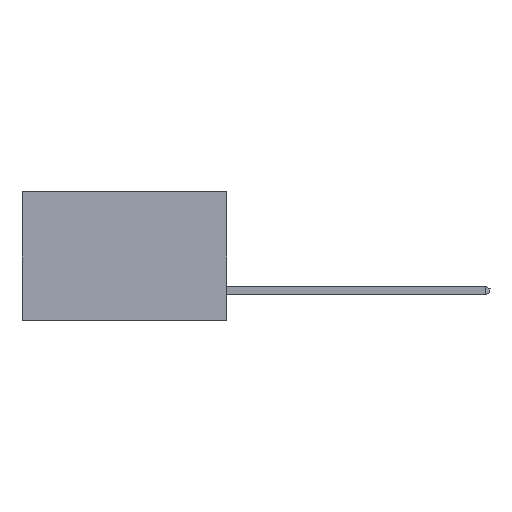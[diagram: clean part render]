
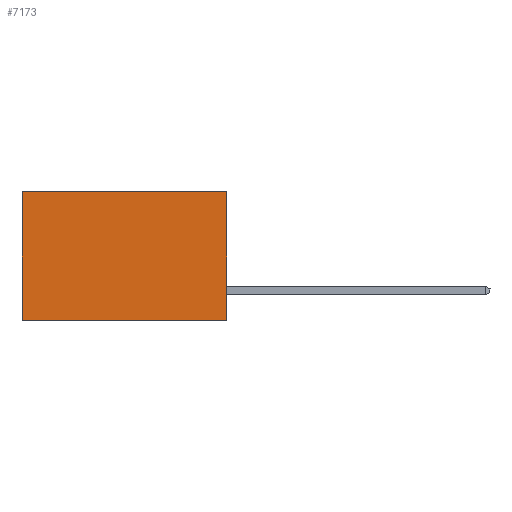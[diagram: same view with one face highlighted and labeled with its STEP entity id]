
A CAD part, left-side view. The second image highlights one B-rep face of the part: STEP entity #7173.
In plain terms, the highlighted planar face has unit normal (-1, 0, 0).
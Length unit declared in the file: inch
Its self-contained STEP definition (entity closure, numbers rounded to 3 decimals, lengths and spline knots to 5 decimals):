
#191 = DIRECTION ( 'NONE',  ( 0., 0., -1. ) ) ;
#784 = ORIENTED_EDGE ( 'NONE', *, *, #5663, .F. ) ;
#1649 = EDGE_CURVE ( 'NONE', #17510, #7373, #10365, .T. ) ;
#2158 = CARTESIAN_POINT ( 'NONE',  ( 0.277, 0., 0. ) ) ;
#2468 = LINE ( 'NONE', #11573, #13204 ) ;
#2965 = DIRECTION ( 'NONE',  ( 0., 1., 0. ) ) ;
#3999 = VECTOR ( 'NONE', #13359, 39.37008 ) ;
#4434 = LINE ( 'NONE', #2158, #3999 ) ;
#4479 = ORIENTED_EDGE ( 'NONE', *, *, #17605, .T. ) ;
#4794 = CARTESIAN_POINT ( 'NONE',  ( 0.277, 0., -0.37 ) ) ;
#5663 = EDGE_CURVE ( 'NONE', #14121, #17510, #2468, .T. ) ;
#7173 = ADVANCED_FACE ( 'NONE', ( #14217 ), #11836, .F. ) ;
#7373 = VERTEX_POINT ( 'NONE', #9023 ) ;
#8032 = EDGE_LOOP ( 'NONE', ( #16727, #12455, #784, #4479 ) ) ;
#9023 = CARTESIAN_POINT ( 'NONE',  ( 0.277, 0.59, -0.37 ) ) ;
#9721 = AXIS2_PLACEMENT_3D ( 'NONE', #12255, #11832, #11819 ) ;
#10365 = LINE ( 'NONE', #4794, #13638 ) ;
#11429 = CARTESIAN_POINT ( 'NONE',  ( 0.277, 0., 0. ) ) ;
#11532 = CARTESIAN_POINT ( 'NONE',  ( 0.277, 0.59, 0. ) ) ;
#11573 = CARTESIAN_POINT ( 'NONE',  ( 0.277, 0., -0.37 ) ) ;
#11819 = DIRECTION ( 'NONE',  ( 0., 0., -1. ) ) ;
#11832 = DIRECTION ( 'NONE',  ( 1., 0., 0. ) ) ;
#11836 = PLANE ( 'NONE',  #9721 ) ;
#11979 = VECTOR ( 'NONE', #191, 39.37008 ) ;
#12255 = CARTESIAN_POINT ( 'NONE',  ( 0.277, 0., -0.37 ) ) ;
#12455 = ORIENTED_EDGE ( 'NONE', *, *, #1649, .F. ) ;
#12848 = CARTESIAN_POINT ( 'NONE',  ( 0.277, 0.59, -0.37 ) ) ;
#13204 = VECTOR ( 'NONE', #14391, 39.37008 ) ;
#13359 = DIRECTION ( 'NONE',  ( 0., 1., 0. ) ) ;
#13405 = VERTEX_POINT ( 'NONE', #11532 ) ;
#13638 = VECTOR ( 'NONE', #2965, 39.37008 ) ;
#14121 = VERTEX_POINT ( 'NONE', #11429 ) ;
#14217 = FACE_OUTER_BOUND ( 'NONE', #8032, .T. ) ;
#14391 = DIRECTION ( 'NONE',  ( 0., 0., -1. ) ) ;
#15617 = LINE ( 'NONE', #12848, #11979 ) ;
#15900 = EDGE_CURVE ( 'NONE', #13405, #7373, #15617, .T. ) ;
#16727 = ORIENTED_EDGE ( 'NONE', *, *, #15900, .T. ) ;
#17219 = CARTESIAN_POINT ( 'NONE',  ( 0.277, 0., -0.37 ) ) ;
#17510 = VERTEX_POINT ( 'NONE', #17219 ) ;
#17605 = EDGE_CURVE ( 'NONE', #14121, #13405, #4434, .T. ) ;
